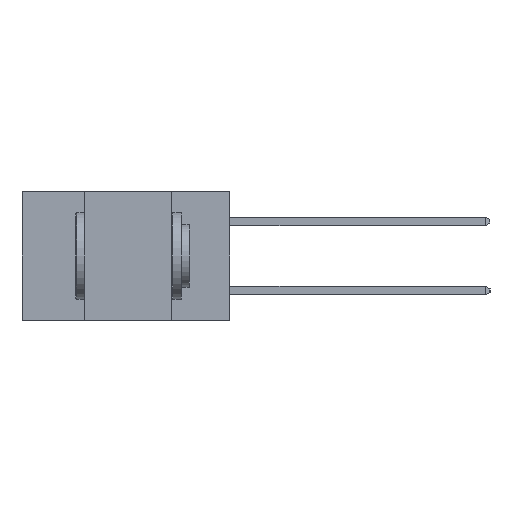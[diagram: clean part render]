
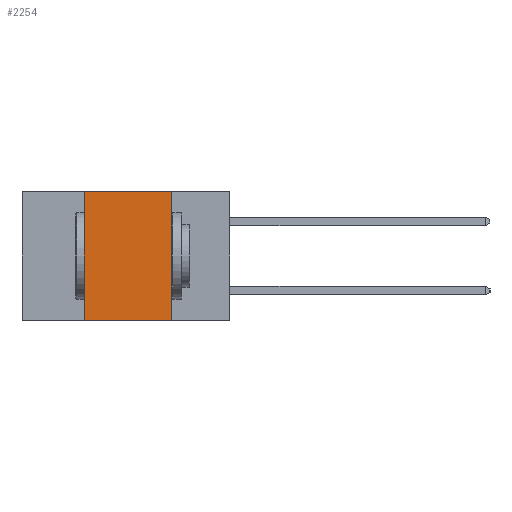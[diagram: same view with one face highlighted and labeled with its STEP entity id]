
A CAD part, left-side view. The second image highlights one B-rep face of the part: STEP entity #2254.
In plain terms, the highlighted planar face has unit normal (-1, 0, 0).
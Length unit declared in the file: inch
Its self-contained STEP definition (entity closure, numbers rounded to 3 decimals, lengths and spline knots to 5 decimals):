
#274 = DIRECTION ( 'NONE',  ( 0., -1., 0. ) ) ;
#432 = VERTEX_POINT ( 'NONE', #6209 ) ;
#667 = EDGE_CURVE ( 'NONE', #432, #7249, #1013, .T. ) ;
#946 = LINE ( 'NONE', #2421, #11397 ) ;
#1013 = LINE ( 'NONE', #2266, #14570 ) ;
#1237 = DIRECTION ( 'NONE',  ( 0., -1., 0. ) ) ;
#1319 = EDGE_CURVE ( 'NONE', #6767, #1645, #1442, .T. ) ;
#1442 = LINE ( 'NONE', #10696, #15772 ) ;
#1645 = VERTEX_POINT ( 'NONE', #13246 ) ;
#1842 = FACE_OUTER_BOUND ( 'NONE', #5057, .T. ) ;
#2254 = ADVANCED_FACE ( 'NONE', ( #1842 ), #8147, .F. ) ;
#2266 = CARTESIAN_POINT ( 'NONE',  ( 0., 0.6, -0.37 ) ) ;
#2421 = CARTESIAN_POINT ( 'NONE',  ( 0., 0.17, -0.37 ) ) ;
#2936 = CARTESIAN_POINT ( 'NONE',  ( 0., 0.42, 0. ) ) ;
#5041 = EDGE_CURVE ( 'NONE', #432, #6767, #8219, .T. ) ;
#5057 = EDGE_LOOP ( 'NONE', ( #5700, #15997, #5262, #12132 ) ) ;
#5262 = ORIENTED_EDGE ( 'NONE', *, *, #5041, .F. ) ;
#5700 = ORIENTED_EDGE ( 'NONE', *, *, #15998, .F. ) ;
#6209 = CARTESIAN_POINT ( 'NONE',  ( 0., 0.42, -0.37 ) ) ;
#6767 = VERTEX_POINT ( 'NONE', #2936 ) ;
#7244 = DIRECTION ( 'NONE',  ( 0., 0., -1. ) ) ;
#7249 = VERTEX_POINT ( 'NONE', #16155 ) ;
#7799 = VECTOR ( 'NONE', #14934, 39.37008 ) ;
#8000 = DIRECTION ( 'NONE',  ( 1., 0., 0. ) ) ;
#8147 = PLANE ( 'NONE',  #13316 ) ;
#8219 = LINE ( 'NONE', #15602, #7799 ) ;
#10666 = DIRECTION ( 'NONE',  ( 0., 0., -1. ) ) ;
#10696 = CARTESIAN_POINT ( 'NONE',  ( 0., 0.6, 0. ) ) ;
#11397 = VECTOR ( 'NONE', #10666, 39.37008 ) ;
#12132 = ORIENTED_EDGE ( 'NONE', *, *, #667, .T. ) ;
#13246 = CARTESIAN_POINT ( 'NONE',  ( 0., 0.17, 0. ) ) ;
#13316 = AXIS2_PLACEMENT_3D ( 'NONE', #17137, #8000, #7244 ) ;
#14570 = VECTOR ( 'NONE', #274, 39.37008 ) ;
#14934 = DIRECTION ( 'NONE',  ( 0., 0., 1. ) ) ;
#15602 = CARTESIAN_POINT ( 'NONE',  ( 0., 0.42, -0.37 ) ) ;
#15772 = VECTOR ( 'NONE', #1237, 39.37008 ) ;
#15997 = ORIENTED_EDGE ( 'NONE', *, *, #1319, .F. ) ;
#15998 = EDGE_CURVE ( 'NONE', #1645, #7249, #946, .T. ) ;
#16155 = CARTESIAN_POINT ( 'NONE',  ( 0., 0.17, -0.37 ) ) ;
#17137 = CARTESIAN_POINT ( 'NONE',  ( 0., 0.6, 0. ) ) ;
